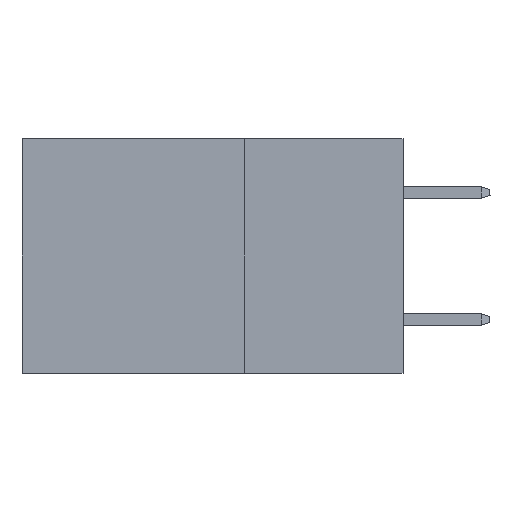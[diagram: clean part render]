
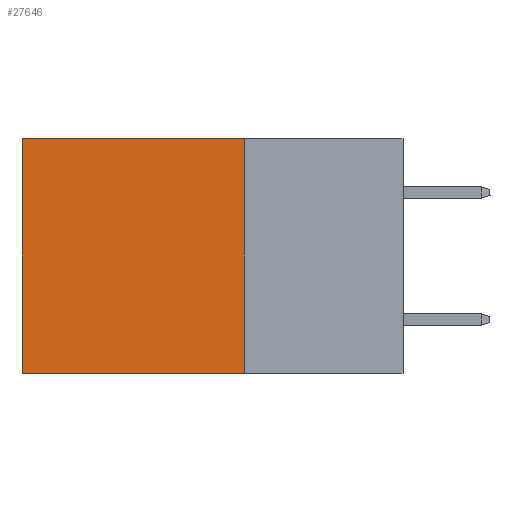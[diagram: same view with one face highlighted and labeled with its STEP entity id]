
A CAD part, left-side view. The second image highlights one B-rep face of the part: STEP entity #27646.
In plain terms, the highlighted planar face has unit normal (-1, 0, 0).
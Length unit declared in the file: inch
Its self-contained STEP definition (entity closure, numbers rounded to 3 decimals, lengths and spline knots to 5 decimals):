
#3926 = CARTESIAN_POINT ( 'NONE',  ( 0.2875, 0.25, -0.37 ) ) ;
#3965 = EDGE_LOOP ( 'NONE', ( #30826, #23527, #34930, #11196 ) ) ;
#5119 = CARTESIAN_POINT ( 'NONE',  ( 0.2875, 0.6, 0. ) ) ;
#6910 = DIRECTION ( 'NONE',  ( 0., 0., -1. ) ) ;
#7082 = VECTOR ( 'NONE', #6910, 39.37008 ) ;
#7128 = CARTESIAN_POINT ( 'NONE',  ( 0.2875, 0.25, 0. ) ) ;
#7545 = LINE ( 'NONE', #7128, #7082 ) ;
#9219 = EDGE_CURVE ( 'NONE', #33191, #14418, #37008, .T. ) ;
#9637 = DIRECTION ( 'NONE',  ( 0., 0., -1. ) ) ;
#11196 = ORIENTED_EDGE ( 'NONE', *, *, #26769, .T. ) ;
#12657 = CARTESIAN_POINT ( 'NONE',  ( 0.2875, 0.25, 0. ) ) ;
#13838 = DIRECTION ( 'NONE',  ( 0., 1., 0. ) ) ;
#14418 = VERTEX_POINT ( 'NONE', #28917 ) ;
#14820 = LINE ( 'NONE', #5119, #39513 ) ;
#15077 = EDGE_CURVE ( 'NONE', #27326, #33191, #7545, .T. ) ;
#15687 = EDGE_CURVE ( 'NONE', #19553, #14418, #14820, .T. ) ;
#16257 = VECTOR ( 'NONE', #13838, 39.37008 ) ;
#18792 = CARTESIAN_POINT ( 'NONE',  ( 0.2875, 0.25, 0. ) ) ;
#19553 = VERTEX_POINT ( 'NONE', #42102 ) ;
#23527 = ORIENTED_EDGE ( 'NONE', *, *, #9219, .F. ) ;
#24580 = CARTESIAN_POINT ( 'NONE',  ( 0.2875, 0.25, -0.37 ) ) ;
#25257 = DIRECTION ( 'NONE',  ( 1., 0., 0. ) ) ;
#26769 = EDGE_CURVE ( 'NONE', #27326, #19553, #29253, .T. ) ;
#26987 = AXIS2_PLACEMENT_3D ( 'NONE', #12657, #25257, #9637 ) ;
#27326 = VERTEX_POINT ( 'NONE', #18792 ) ;
#27646 = ADVANCED_FACE ( 'NONE', ( #35629 ), #42275, .F. ) ;
#28494 = DIRECTION ( 'NONE',  ( 0., 0., -1. ) ) ;
#28917 = CARTESIAN_POINT ( 'NONE',  ( 0.2875, 0.6, -0.37 ) ) ;
#29253 = LINE ( 'NONE', #36159, #39345 ) ;
#29685 = DIRECTION ( 'NONE',  ( 0., 1., 0. ) ) ;
#30826 = ORIENTED_EDGE ( 'NONE', *, *, #15687, .T. ) ;
#33191 = VERTEX_POINT ( 'NONE', #24580 ) ;
#34930 = ORIENTED_EDGE ( 'NONE', *, *, #15077, .F. ) ;
#35629 = FACE_OUTER_BOUND ( 'NONE', #3965, .T. ) ;
#36159 = CARTESIAN_POINT ( 'NONE',  ( 0.2875, 0.25, 0. ) ) ;
#37008 = LINE ( 'NONE', #3926, #16257 ) ;
#39345 = VECTOR ( 'NONE', #29685, 39.37008 ) ;
#39513 = VECTOR ( 'NONE', #28494, 39.37008 ) ;
#42102 = CARTESIAN_POINT ( 'NONE',  ( 0.2875, 0.6, 0. ) ) ;
#42275 = PLANE ( 'NONE',  #26987 ) ;
